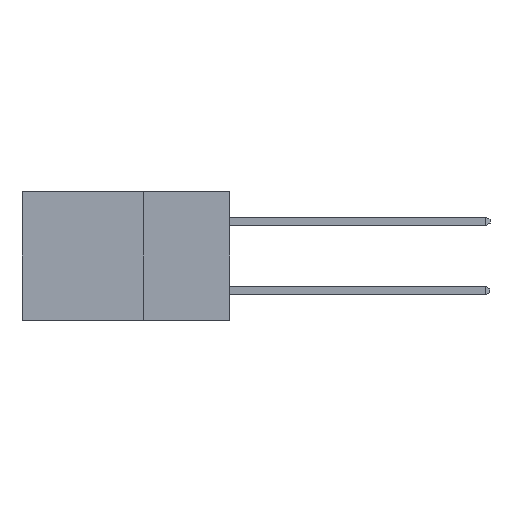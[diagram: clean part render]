
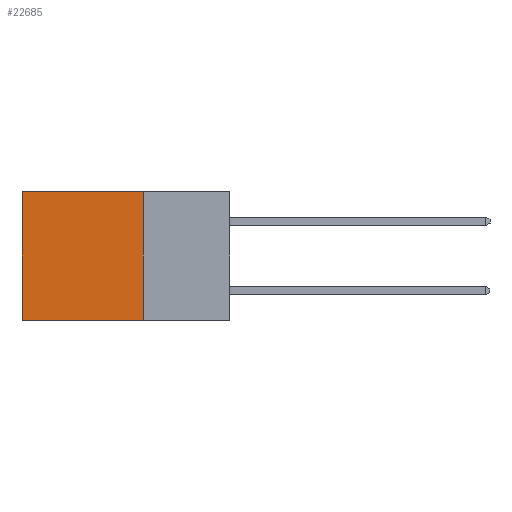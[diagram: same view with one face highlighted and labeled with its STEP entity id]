
A CAD part, left-side view. The second image highlights one B-rep face of the part: STEP entity #22685.
In plain terms, the highlighted planar face has unit normal (-1, 0, 0).
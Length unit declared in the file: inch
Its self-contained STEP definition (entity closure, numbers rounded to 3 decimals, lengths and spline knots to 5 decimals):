
#952 = LINE ( 'NONE', #25117, #11479 ) ;
#1641 = CARTESIAN_POINT ( 'NONE',  ( 0.298, 0.25, 0. ) ) ;
#1795 = VERTEX_POINT ( 'NONE', #2043 ) ;
#2043 = CARTESIAN_POINT ( 'NONE',  ( 0.298, 0.6, 0. ) ) ;
#2172 = DIRECTION ( 'NONE',  ( 0., 1., 0. ) ) ;
#2513 = VECTOR ( 'NONE', #2172, 39.37008 ) ;
#3128 = VERTEX_POINT ( 'NONE', #5029 ) ;
#5029 = CARTESIAN_POINT ( 'NONE',  ( 0.298, 0.25, -0.37 ) ) ;
#5181 = EDGE_CURVE ( 'NONE', #6442, #3128, #952, .T. ) ;
#5959 = ORIENTED_EDGE ( 'NONE', *, *, #25726, .T. ) ;
#5997 = PLANE ( 'NONE',  #8412 ) ;
#6442 = VERTEX_POINT ( 'NONE', #25096 ) ;
#8412 = AXIS2_PLACEMENT_3D ( 'NONE', #12334, #26602, #14425 ) ;
#10349 = ORIENTED_EDGE ( 'NONE', *, *, #14852, .T. ) ;
#11106 = ORIENTED_EDGE ( 'NONE', *, *, #5181, .F. ) ;
#11479 = VECTOR ( 'NONE', #13897, 39.37008 ) ;
#12064 = LINE ( 'NONE', #1641, #22359 ) ;
#12334 = CARTESIAN_POINT ( 'NONE',  ( 0.298, 0.25, 0. ) ) ;
#12843 = CARTESIAN_POINT ( 'NONE',  ( 0.298, 0.6, -0.37 ) ) ;
#13697 = LINE ( 'NONE', #14745, #2513 ) ;
#13897 = DIRECTION ( 'NONE',  ( 0., 0., -1. ) ) ;
#14314 = ORIENTED_EDGE ( 'NONE', *, *, #15000, .F. ) ;
#14425 = DIRECTION ( 'NONE',  ( 0., 0., -1. ) ) ;
#14745 = CARTESIAN_POINT ( 'NONE',  ( 0.298, 0.25, -0.37 ) ) ;
#14852 = EDGE_CURVE ( 'NONE', #6442, #1795, #12064, .T. ) ;
#15000 = EDGE_CURVE ( 'NONE', #3128, #19981, #13697, .T. ) ;
#15490 = CARTESIAN_POINT ( 'NONE',  ( 0.298, 0.6, 0. ) ) ;
#19540 = DIRECTION ( 'NONE',  ( 0., 0., -1. ) ) ;
#19765 = FACE_OUTER_BOUND ( 'NONE', #21097, .T. ) ;
#19981 = VERTEX_POINT ( 'NONE', #12843 ) ;
#21097 = EDGE_LOOP ( 'NONE', ( #5959, #14314, #11106, #10349 ) ) ;
#22359 = VECTOR ( 'NONE', #22452, 39.37008 ) ;
#22452 = DIRECTION ( 'NONE',  ( 0., 1., 0. ) ) ;
#22685 = ADVANCED_FACE ( 'NONE', ( #19765 ), #5997, .F. ) ;
#24008 = VECTOR ( 'NONE', #19540, 39.37008 ) ;
#24635 = LINE ( 'NONE', #15490, #24008 ) ;
#25096 = CARTESIAN_POINT ( 'NONE',  ( 0.298, 0.25, 0. ) ) ;
#25117 = CARTESIAN_POINT ( 'NONE',  ( 0.298, 0.25, 0. ) ) ;
#25726 = EDGE_CURVE ( 'NONE', #1795, #19981, #24635, .T. ) ;
#26602 = DIRECTION ( 'NONE',  ( 1., 0., 0. ) ) ;
